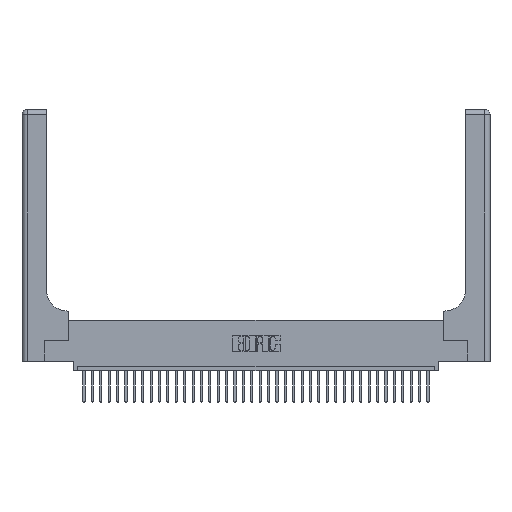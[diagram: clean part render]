
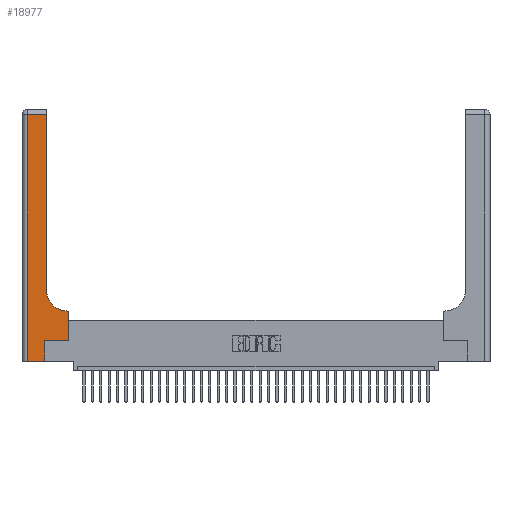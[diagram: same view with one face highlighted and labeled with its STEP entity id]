
A CAD part, top view. The second image highlights one B-rep face of the part: STEP entity #18977.
In plain terms, the highlighted planar face has unit normal (0, 0, 1).
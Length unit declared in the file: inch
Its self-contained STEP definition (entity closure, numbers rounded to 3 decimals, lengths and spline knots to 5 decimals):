
#69 = DIRECTION ( 'NONE',  ( 1., 0., 0. ) ) ;
#962 = DIRECTION ( 'NONE',  ( -1., 0., 0. ) ) ;
#1705 = CARTESIAN_POINT ( 'NONE',  ( 0.2915, 3., 0.37 ) ) ;
#1840 = CARTESIAN_POINT ( 'NONE',  ( 0.5585, 0.25, 0.37 ) ) ;
#2103 = DIRECTION ( 'NONE',  ( 0., 0., -1. ) ) ;
#2679 = CARTESIAN_POINT ( 'NONE',  ( 0.269, 0.25, 0.37 ) ) ;
#2751 = VERTEX_POINT ( 'NONE', #9852 ) ;
#3152 = LINE ( 'NONE', #1705, #29053 ) ;
#3242 = VECTOR ( 'NONE', #19629, 39.37008 ) ;
#3533 = VERTEX_POINT ( 'NONE', #22723 ) ;
#3635 = CARTESIAN_POINT ( 'NONE',  ( 0.2915, 0.85, 0.37 ) ) ;
#3898 = VECTOR ( 'NONE', #11491, 39.37008 ) ;
#3908 = ORIENTED_EDGE ( 'NONE', *, *, #11752, .T. ) ;
#4666 = VERTEX_POINT ( 'NONE', #19759 ) ;
#5181 = CARTESIAN_POINT ( 'NONE',  ( 0.269, 0., 0.37 ) ) ;
#5778 = CARTESIAN_POINT ( 'NONE',  ( 0.5585, 0.6, 0.37 ) ) ;
#5918 = EDGE_CURVE ( 'NONE', #28710, #2751, #30117, .T. ) ;
#5963 = ORIENTED_EDGE ( 'NONE', *, *, #10637, .T. ) ;
#7169 = ORIENTED_EDGE ( 'NONE', *, *, #15591, .T. ) ;
#7474 = VECTOR ( 'NONE', #27278, 39.37008 ) ;
#7648 = ORIENTED_EDGE ( 'NONE', *, *, #33492, .T. ) ;
#7709 = ORIENTED_EDGE ( 'NONE', *, *, #19766, .T. ) ;
#7809 = CARTESIAN_POINT ( 'NONE',  ( 0., 3., 0.37 ) ) ;
#9119 = VECTOR ( 'NONE', #962, 39.37008 ) ;
#9138 = VECTOR ( 'NONE', #36353, 39.37008 ) ;
#9406 = DIRECTION ( 'NONE',  ( 0., 0., -1. ) ) ;
#9852 = CARTESIAN_POINT ( 'NONE',  ( 0.06, 2.94, 0.37 ) ) ;
#9983 = VERTEX_POINT ( 'NONE', #15082 ) ;
#10133 = AXIS2_PLACEMENT_3D ( 'NONE', #7809, #2103, #25799 ) ;
#10637 = EDGE_CURVE ( 'NONE', #23466, #4666, #31115, .T. ) ;
#10789 = LINE ( 'NONE', #16954, #3242 ) ;
#11491 = DIRECTION ( 'NONE',  ( 0., 1., 0. ) ) ;
#11752 = EDGE_CURVE ( 'NONE', #32072, #3533, #27510, .T. ) ;
#13448 = CIRCLE ( 'NONE', #33074, 0.25 ) ;
#14138 = LINE ( 'NONE', #18139, #3898 ) ;
#15082 = CARTESIAN_POINT ( 'NONE',  ( 0.06, 0., 0.37 ) ) ;
#15473 = ORIENTED_EDGE ( 'NONE', *, *, #5918, .T. ) ;
#15591 = EDGE_CURVE ( 'NONE', #4666, #32023, #13448, .T. ) ;
#15885 = CARTESIAN_POINT ( 'NONE',  ( 0.2915, 0.6, 0.37 ) ) ;
#16438 = ORIENTED_EDGE ( 'NONE', *, *, #26202, .T. ) ;
#16697 = LINE ( 'NONE', #1840, #9138 ) ;
#16954 = CARTESIAN_POINT ( 'NONE',  ( 0.06, 3., 0.37 ) ) ;
#17006 = DIRECTION ( 'NONE',  ( 1., 0., 0. ) ) ;
#17769 = CARTESIAN_POINT ( 'NONE',  ( 0.2915, 2.94, 0.37 ) ) ;
#18139 = CARTESIAN_POINT ( 'NONE',  ( 0.269, 0., 0.37 ) ) ;
#18656 = DIRECTION ( 'NONE',  ( 0., 1., 0. ) ) ;
#18977 = ADVANCED_FACE ( 'NONE', ( #35128 ), #21949, .F. ) ;
#19629 = DIRECTION ( 'NONE',  ( 0., -1., 0. ) ) ;
#19759 = CARTESIAN_POINT ( 'NONE',  ( 0.5415, 0.6, 0.37 ) ) ;
#19766 = EDGE_CURVE ( 'NONE', #9983, #21156, #31482, .T. ) ;
#19915 = VECTOR ( 'NONE', #69, 39.37008 ) ;
#21156 = VERTEX_POINT ( 'NONE', #5181 ) ;
#21795 = EDGE_CURVE ( 'NONE', #2751, #9983, #10789, .T. ) ;
#21949 = PLANE ( 'NONE',  #10133 ) ;
#22027 = EDGE_LOOP ( 'NONE', ( #16438, #15473, #36554, #7709, #26753, #3908, #7648, #5963, #7169 ) ) ;
#22723 = CARTESIAN_POINT ( 'NONE',  ( 0.5585, 0.25, 0.37 ) ) ;
#23466 = VERTEX_POINT ( 'NONE', #5778 ) ;
#23964 = CARTESIAN_POINT ( 'NONE',  ( 0., 2.94, 0.37 ) ) ;
#25799 = DIRECTION ( 'NONE',  ( -1., 0., 0. ) ) ;
#25987 = CARTESIAN_POINT ( 'NONE',  ( 0.269, 0.25, 0.37 ) ) ;
#26202 = EDGE_CURVE ( 'NONE', #32023, #28710, #3152, .T. ) ;
#26753 = ORIENTED_EDGE ( 'NONE', *, *, #27884, .T. ) ;
#27278 = DIRECTION ( 'NONE',  ( -1., 0., 0. ) ) ;
#27510 = LINE ( 'NONE', #2679, #19915 ) ;
#27884 = EDGE_CURVE ( 'NONE', #21156, #32072, #14138, .T. ) ;
#28710 = VERTEX_POINT ( 'NONE', #17769 ) ;
#29053 = VECTOR ( 'NONE', #18656, 39.37008 ) ;
#30117 = LINE ( 'NONE', #23964, #9119 ) ;
#31004 = CARTESIAN_POINT ( 'NONE',  ( 0.5415, 0.85, 0.37 ) ) ;
#31115 = LINE ( 'NONE', #15885, #7474 ) ;
#31482 = LINE ( 'NONE', #36462, #36368 ) ;
#32023 = VERTEX_POINT ( 'NONE', #3635 ) ;
#32072 = VERTEX_POINT ( 'NONE', #25987 ) ;
#33074 = AXIS2_PLACEMENT_3D ( 'NONE', #31004, #9406, #17006 ) ;
#33492 = EDGE_CURVE ( 'NONE', #3533, #23466, #16697, .T. ) ;
#33722 = DIRECTION ( 'NONE',  ( 1., 0., 0. ) ) ;
#35128 = FACE_OUTER_BOUND ( 'NONE', #22027, .T. ) ;
#36353 = DIRECTION ( 'NONE',  ( 0., 1., 0. ) ) ;
#36368 = VECTOR ( 'NONE', #33722, 39.37008 ) ;
#36462 = CARTESIAN_POINT ( 'NONE',  ( 0., 0., 0.37 ) ) ;
#36554 = ORIENTED_EDGE ( 'NONE', *, *, #21795, .T. ) ;
